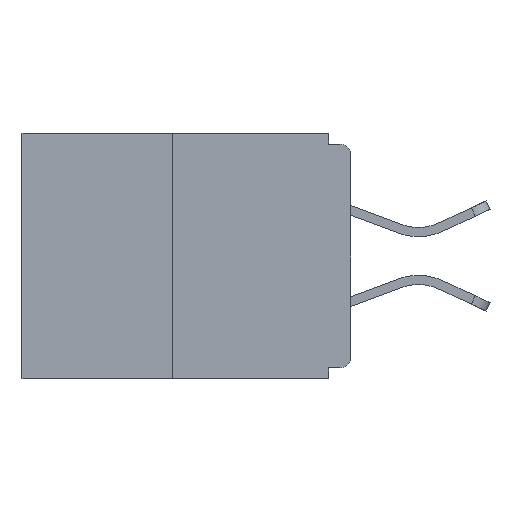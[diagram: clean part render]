
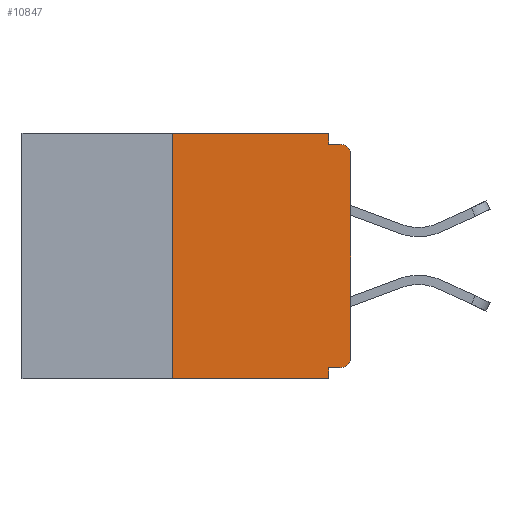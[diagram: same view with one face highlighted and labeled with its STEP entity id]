
A CAD part, left-side view. The second image highlights one B-rep face of the part: STEP entity #10847.
In plain terms, the highlighted planar face has unit normal (-1, 0, 0).
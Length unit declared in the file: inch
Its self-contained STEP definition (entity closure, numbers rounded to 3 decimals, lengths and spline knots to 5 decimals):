
#478 = DIRECTION ( 'NONE',  ( 1., 0., 0. ) ) ;
#635 = DIRECTION ( 'NONE',  ( 0., 0., -1. ) ) ;
#970 = VERTEX_POINT ( 'NONE', #7263 ) ;
#1035 = AXIS2_PLACEMENT_3D ( 'NONE', #15851, #2913, #6381 ) ;
#1174 = EDGE_CURVE ( 'NONE', #970, #3903, #5751, .T. ) ;
#1289 = VERTEX_POINT ( 'NONE', #18943 ) ;
#1323 = ORIENTED_EDGE ( 'NONE', *, *, #1174, .F. ) ;
#1449 = VECTOR ( 'NONE', #2733, 39.37008 ) ;
#1671 = DIRECTION ( 'NONE',  ( 0., -1., 0. ) ) ;
#1824 = CARTESIAN_POINT ( 'NONE',  ( 0., 0.46, 0. ) ) ;
#2089 = EDGE_CURVE ( 'NONE', #12879, #11531, #9413, .T. ) ;
#2242 = CARTESIAN_POINT ( 'NONE',  ( 0., 0.46, 0. ) ) ;
#2307 = VECTOR ( 'NONE', #12882, 39.37008 ) ;
#2733 = DIRECTION ( 'NONE',  ( 0., 0., 1. ) ) ;
#2913 = DIRECTION ( 'NONE',  ( -1., 0., 0. ) ) ;
#3903 = VERTEX_POINT ( 'NONE', #12775 ) ;
#4380 = LINE ( 'NONE', #10621, #7162 ) ;
#4596 = VERTEX_POINT ( 'NONE', #5455 ) ;
#4611 = ORIENTED_EDGE ( 'NONE', *, *, #7674, .T. ) ;
#4713 = CARTESIAN_POINT ( 'NONE',  ( 0., 0., -0.03 ) ) ;
#5039 = ORIENTED_EDGE ( 'NONE', *, *, #6058, .T. ) ;
#5408 = VECTOR ( 'NONE', #1671, 39.37008 ) ;
#5424 = PLANE ( 'NONE',  #20588 ) ;
#5455 = CARTESIAN_POINT ( 'NONE',  ( 0., 0., -0.313 ) ) ;
#5751 = LINE ( 'NONE', #1824, #7287 ) ;
#5982 = LINE ( 'NONE', #7604, #1449 ) ;
#6058 = EDGE_CURVE ( 'NONE', #18131, #1289, #7253, .T. ) ;
#6381 = DIRECTION ( 'NONE',  ( 0., 0., -1. ) ) ;
#6484 = ORIENTED_EDGE ( 'NONE', *, *, #13706, .F. ) ;
#6984 = FACE_OUTER_BOUND ( 'NONE', #11354, .T. ) ;
#7048 = CARTESIAN_POINT ( 'NONE',  ( 0., 0.031, -0.343 ) ) ;
#7162 = VECTOR ( 'NONE', #12258, 39.37008 ) ;
#7253 = CIRCLE ( 'NONE', #1035, 0.015 ) ;
#7263 = CARTESIAN_POINT ( 'NONE',  ( 0., 0.25, 0. ) ) ;
#7283 = DIRECTION ( 'NONE',  ( 0., 1., 0. ) ) ;
#7287 = VECTOR ( 'NONE', #11413, 39.37008 ) ;
#7604 = CARTESIAN_POINT ( 'NONE',  ( 0., 0.25, 0. ) ) ;
#7674 = EDGE_CURVE ( 'NONE', #19586, #17735, #4380, .T. ) ;
#7754 = DIRECTION ( 'NONE',  ( -1., 0., 0. ) ) ;
#7901 = CARTESIAN_POINT ( 'NONE',  ( 0., 0.015, -0.328 ) ) ;
#8405 = VECTOR ( 'NONE', #7283, 39.37008 ) ;
#8530 = CARTESIAN_POINT ( 'NONE',  ( 0., 0.031, -0.343 ) ) ;
#9105 = EDGE_CURVE ( 'NONE', #4596, #18131, #19174, .T. ) ;
#9116 = CARTESIAN_POINT ( 'NONE',  ( 0., 0., 0. ) ) ;
#9413 = LINE ( 'NONE', #15482, #8405 ) ;
#9598 = VECTOR ( 'NONE', #635, 39.37008 ) ;
#9684 = CIRCLE ( 'NONE', #18434, 0.015 ) ;
#9831 = VECTOR ( 'NONE', #10731, 39.37008 ) ;
#9965 = EDGE_CURVE ( 'NONE', #19586, #970, #5982, .T. ) ;
#10248 = ORIENTED_EDGE ( 'NONE', *, *, #18676, .T. ) ;
#10621 = CARTESIAN_POINT ( 'NONE',  ( 0., 0.46, -0.343 ) ) ;
#10731 = DIRECTION ( 'NONE',  ( 0., 0., 1. ) ) ;
#10837 = LINE ( 'NONE', #7048, #9598 ) ;
#10847 = ADVANCED_FACE ( 'NONE', ( #6984 ), #5424, .F. ) ;
#11354 = EDGE_LOOP ( 'NONE', ( #1323, #19143, #4611, #17852, #13435, #10248, #16947, #5039, #13587, #6484 ) ) ;
#11413 = DIRECTION ( 'NONE',  ( 0., -1., 0. ) ) ;
#11500 = CARTESIAN_POINT ( 'NONE',  ( 0., 0.031, -0.015 ) ) ;
#11531 = VERTEX_POINT ( 'NONE', #13663 ) ;
#12258 = DIRECTION ( 'NONE',  ( 0., -1., 0. ) ) ;
#12320 = VERTEX_POINT ( 'NONE', #11500 ) ;
#12498 = EDGE_CURVE ( 'NONE', #12320, #1289, #14766, .T. ) ;
#12775 = CARTESIAN_POINT ( 'NONE',  ( 0., 0.031, 0. ) ) ;
#12879 = VERTEX_POINT ( 'NONE', #7901 ) ;
#12882 = DIRECTION ( 'NONE',  ( 0., 0., -1. ) ) ;
#13321 = CARTESIAN_POINT ( 'NONE',  ( 0., 0.25, -0.343 ) ) ;
#13435 = ORIENTED_EDGE ( 'NONE', *, *, #2089, .F. ) ;
#13587 = ORIENTED_EDGE ( 'NONE', *, *, #12498, .F. ) ;
#13663 = CARTESIAN_POINT ( 'NONE',  ( 0., 0.031, -0.328 ) ) ;
#13706 = EDGE_CURVE ( 'NONE', #3903, #12320, #18258, .T. ) ;
#14464 = CARTESIAN_POINT ( 'NONE',  ( 0., 0., -0.015 ) ) ;
#14766 = LINE ( 'NONE', #14464, #5408 ) ;
#15198 = EDGE_CURVE ( 'NONE', #11531, #17735, #10837, .T. ) ;
#15482 = CARTESIAN_POINT ( 'NONE',  ( 0., 0., -0.328 ) ) ;
#15851 = CARTESIAN_POINT ( 'NONE',  ( 0., 0.015, -0.03 ) ) ;
#16947 = ORIENTED_EDGE ( 'NONE', *, *, #9105, .T. ) ;
#17443 = CARTESIAN_POINT ( 'NONE',  ( 0., 0.015, -0.313 ) ) ;
#17735 = VERTEX_POINT ( 'NONE', #8530 ) ;
#17852 = ORIENTED_EDGE ( 'NONE', *, *, #15198, .F. ) ;
#18060 = CARTESIAN_POINT ( 'NONE',  ( 0., 0.031, 0. ) ) ;
#18131 = VERTEX_POINT ( 'NONE', #4713 ) ;
#18258 = LINE ( 'NONE', #18060, #2307 ) ;
#18434 = AXIS2_PLACEMENT_3D ( 'NONE', #17443, #7754, #19051 ) ;
#18435 = DIRECTION ( 'NONE',  ( 0., 0., -1. ) ) ;
#18676 = EDGE_CURVE ( 'NONE', #12879, #4596, #9684, .T. ) ;
#18943 = CARTESIAN_POINT ( 'NONE',  ( 0., 0.015, -0.015 ) ) ;
#19051 = DIRECTION ( 'NONE',  ( 0., 0., -1. ) ) ;
#19143 = ORIENTED_EDGE ( 'NONE', *, *, #9965, .F. ) ;
#19174 = LINE ( 'NONE', #9116, #9831 ) ;
#19586 = VERTEX_POINT ( 'NONE', #13321 ) ;
#20588 = AXIS2_PLACEMENT_3D ( 'NONE', #2242, #478, #18435 ) ;
